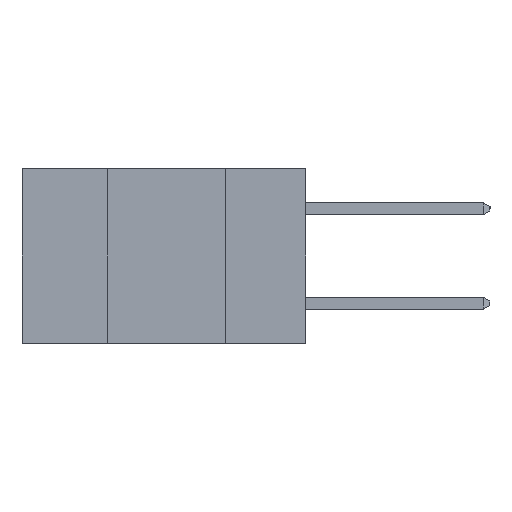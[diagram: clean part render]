
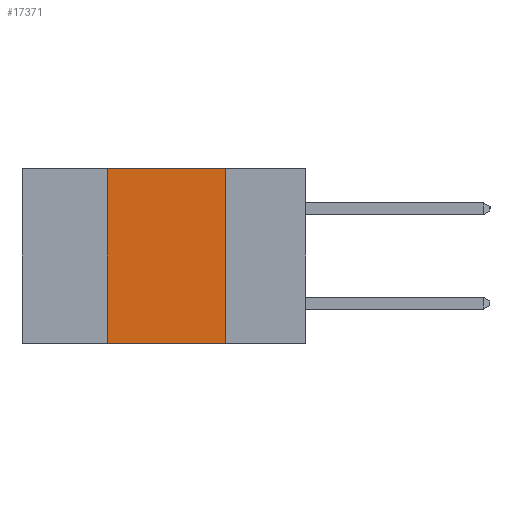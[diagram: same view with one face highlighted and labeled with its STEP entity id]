
A CAD part, left-side view. The second image highlights one B-rep face of the part: STEP entity #17371.
In plain terms, the highlighted planar face has unit normal (-1, 0, 0).
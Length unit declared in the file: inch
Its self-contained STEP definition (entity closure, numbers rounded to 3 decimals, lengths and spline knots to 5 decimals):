
#886 = EDGE_CURVE ( 'NONE', #12812, #9968, #10111, .T. ) ;
#2049 = EDGE_CURVE ( 'NONE', #21909, #12812, #17836, .T. ) ;
#2141 = FACE_OUTER_BOUND ( 'NONE', #4901, .T. ) ;
#3128 = ORIENTED_EDGE ( 'NONE', *, *, #11328, .F. ) ;
#3300 = CARTESIAN_POINT ( 'NONE',  ( 0., 0.42, -0.37 ) ) ;
#3705 = CARTESIAN_POINT ( 'NONE',  ( 0., 0.17, -0.37 ) ) ;
#3981 = CARTESIAN_POINT ( 'NONE',  ( 0., 0.42, 0. ) ) ;
#4107 = DIRECTION ( 'NONE',  ( 0., -1., 0. ) ) ;
#4901 = EDGE_LOOP ( 'NONE', ( #19086, #17467, #3128, #16306 ) ) ;
#5593 = CARTESIAN_POINT ( 'NONE',  ( 0., 0.17, 0. ) ) ;
#5598 = PLANE ( 'NONE',  #10422 ) ;
#6841 = DIRECTION ( 'NONE',  ( 0., -1., 0. ) ) ;
#7112 = DIRECTION ( 'NONE',  ( 0., 0., 1. ) ) ;
#7723 = EDGE_CURVE ( 'NONE', #11127, #9968, #11617, .T. ) ;
#7775 = VECTOR ( 'NONE', #22795, 39.37008 ) ;
#8278 = VECTOR ( 'NONE', #4107, 39.37008 ) ;
#9968 = VERTEX_POINT ( 'NONE', #3705 ) ;
#10111 = LINE ( 'NONE', #10340, #7775 ) ;
#10340 = CARTESIAN_POINT ( 'NONE',  ( 0., 0.17, -0.37 ) ) ;
#10422 = AXIS2_PLACEMENT_3D ( 'NONE', #18397, #16477, #14313 ) ;
#11127 = VERTEX_POINT ( 'NONE', #3300 ) ;
#11328 = EDGE_CURVE ( 'NONE', #11127, #21909, #16086, .T. ) ;
#11617 = LINE ( 'NONE', #15450, #8278 ) ;
#12812 = VERTEX_POINT ( 'NONE', #5593 ) ;
#12849 = CARTESIAN_POINT ( 'NONE',  ( 0., 0.42, -0.37 ) ) ;
#14313 = DIRECTION ( 'NONE',  ( 0., 0., -1. ) ) ;
#14474 = VECTOR ( 'NONE', #7112, 39.37008 ) ;
#15450 = CARTESIAN_POINT ( 'NONE',  ( 0., 0.6, -0.37 ) ) ;
#16086 = LINE ( 'NONE', #12849, #14474 ) ;
#16306 = ORIENTED_EDGE ( 'NONE', *, *, #7723, .T. ) ;
#16477 = DIRECTION ( 'NONE',  ( 1., 0., 0. ) ) ;
#17371 = ADVANCED_FACE ( 'NONE', ( #2141 ), #5598, .F. ) ;
#17467 = ORIENTED_EDGE ( 'NONE', *, *, #2049, .F. ) ;
#17836 = LINE ( 'NONE', #23586, #20724 ) ;
#18397 = CARTESIAN_POINT ( 'NONE',  ( 0., 0.6, 0. ) ) ;
#19086 = ORIENTED_EDGE ( 'NONE', *, *, #886, .F. ) ;
#20724 = VECTOR ( 'NONE', #6841, 39.37008 ) ;
#21909 = VERTEX_POINT ( 'NONE', #3981 ) ;
#22795 = DIRECTION ( 'NONE',  ( 0., 0., -1. ) ) ;
#23586 = CARTESIAN_POINT ( 'NONE',  ( 0., 0.6, 0. ) ) ;
